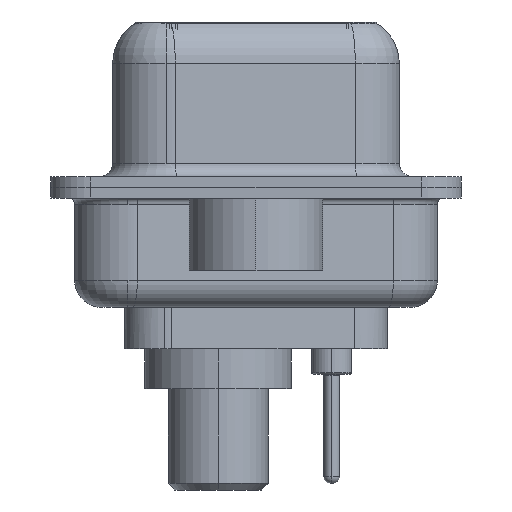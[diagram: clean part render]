
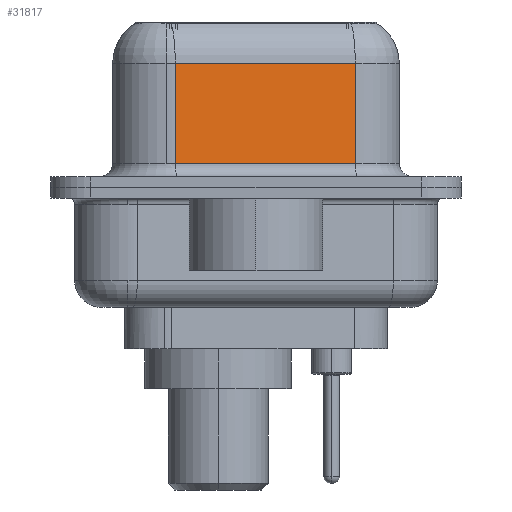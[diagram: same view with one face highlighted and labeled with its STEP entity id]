
A CAD part, left-side view. The second image highlights one B-rep face of the part: STEP entity #31817.
In plain terms, the highlighted planar face has unit normal (-0.985, -0.174, 0).
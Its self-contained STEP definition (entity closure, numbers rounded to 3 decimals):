
#1271 = VERTEX_POINT ( 'NONE', #30869 ) ;
#1444 = VERTEX_POINT ( 'NONE', #3437 ) ;
#1589 = CARTESIAN_POINT ( 'NONE',  ( 5.621, -3.722, 4.65 ) ) ;
#1999 = DIRECTION ( 'NONE',  ( 0., 0., -1. ) ) ;
#3437 = CARTESIAN_POINT ( 'NONE',  ( 5.621, -3.722, 4.65 ) ) ;
#4823 = VERTEX_POINT ( 'NONE', #13510 ) ;
#5581 = PLANE ( 'NONE',  #20355 ) ;
#6231 = LINE ( 'NONE', #1589, #32160 ) ;
#6472 = VECTOR ( 'NONE', #1999, 1000. ) ;
#6857 = EDGE_CURVE ( 'NONE', #4823, #1271, #16284, .T. ) ;
#6954 = EDGE_CURVE ( 'NONE', #1444, #1271, #20592, .T. ) ;
#8131 = ORIENTED_EDGE ( 'NONE', *, *, #6954, .F. ) ;
#8272 = LINE ( 'NONE', #15323, #9838 ) ;
#9838 = VECTOR ( 'NONE', #28400, 1000. ) ;
#11645 = CARTESIAN_POINT ( 'NONE',  ( 5.621, -3.722, 0.9 ) ) ;
#13170 = VERTEX_POINT ( 'NONE', #23689 ) ;
#13510 = CARTESIAN_POINT ( 'NONE',  ( 4.43, 3.028, 0.9 ) ) ;
#14252 = DIRECTION ( 'NONE',  ( 0.174, -0.985, 0. ) ) ;
#15323 = CARTESIAN_POINT ( 'NONE',  ( 4.43, 3.028, 6.4 ) ) ;
#16284 = LINE ( 'NONE', #11645, #22183 ) ;
#17598 = EDGE_CURVE ( 'NONE', #1444, #13170, #6231, .T. ) ;
#20355 = AXIS2_PLACEMENT_3D ( 'NONE', #30485, #23113, #28184 ) ;
#20592 = LINE ( 'NONE', #29543, #6472 ) ;
#20671 = EDGE_LOOP ( 'NONE', ( #8131, #28198, #29530, #29086 ) ) ;
#22183 = VECTOR ( 'NONE', #14252, 1000. ) ;
#23113 = DIRECTION ( 'NONE',  ( 0.985, 0.174, 0. ) ) ;
#23206 = FACE_OUTER_BOUND ( 'NONE', #20671, .T. ) ;
#23412 = EDGE_CURVE ( 'NONE', #13170, #4823, #8272, .T. ) ;
#23689 = CARTESIAN_POINT ( 'NONE',  ( 4.43, 3.028, 4.65 ) ) ;
#28184 = DIRECTION ( 'NONE',  ( -0.174, 0.985, 0. ) ) ;
#28198 = ORIENTED_EDGE ( 'NONE', *, *, #17598, .T. ) ;
#28400 = DIRECTION ( 'NONE',  ( 0., 0., -1. ) ) ;
#29086 = ORIENTED_EDGE ( 'NONE', *, *, #6857, .T. ) ;
#29265 = DIRECTION ( 'NONE',  ( -0.174, 0.985, 0. ) ) ;
#29530 = ORIENTED_EDGE ( 'NONE', *, *, #23412, .T. ) ;
#29543 = CARTESIAN_POINT ( 'NONE',  ( 5.621, -3.722, 6.4 ) ) ;
#30485 = CARTESIAN_POINT ( 'NONE',  ( 5.621, -3.722, 6.4 ) ) ;
#30869 = CARTESIAN_POINT ( 'NONE',  ( 5.621, -3.722, 0.9 ) ) ;
#31817 = ADVANCED_FACE ( 'NONE', ( #23206 ), #5581, .F. ) ;
#32160 = VECTOR ( 'NONE', #29265, 1000. ) ;
